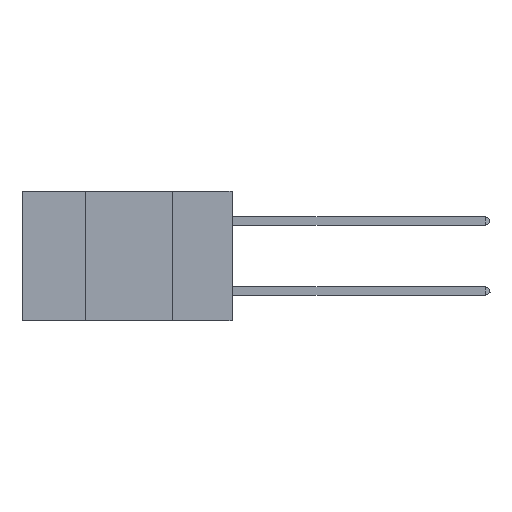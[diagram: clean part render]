
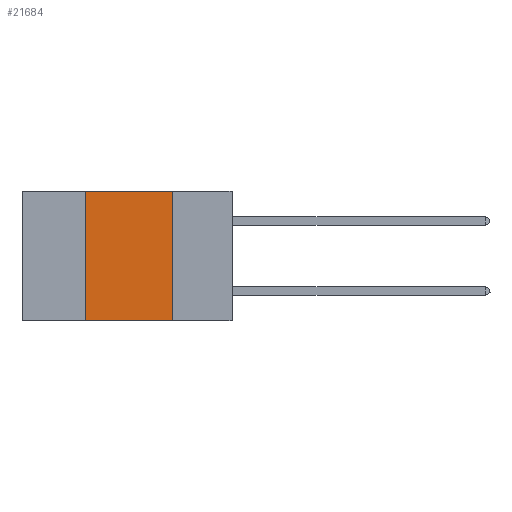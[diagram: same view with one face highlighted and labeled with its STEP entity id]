
A CAD part, left-side view. The second image highlights one B-rep face of the part: STEP entity #21684.
In plain terms, the highlighted planar face has unit normal (-1, 0, 0).
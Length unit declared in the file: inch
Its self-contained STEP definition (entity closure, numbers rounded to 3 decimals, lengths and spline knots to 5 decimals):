
#92 = CARTESIAN_POINT ( 'NONE',  ( 0., 0.42, 0. ) ) ;
#700 = AXIS2_PLACEMENT_3D ( 'NONE', #7568, #22101, #24284 ) ;
#1999 = DIRECTION ( 'NONE',  ( 0., -1., 0. ) ) ;
#3115 = EDGE_CURVE ( 'NONE', #4503, #23749, #26692, .T. ) ;
#3599 = EDGE_CURVE ( 'NONE', #7550, #9196, #25687, .T. ) ;
#3965 = EDGE_LOOP ( 'NONE', ( #4699, #14611, #3979, #21877 ) ) ;
#3979 = ORIENTED_EDGE ( 'NONE', *, *, #16165, .F. ) ;
#4019 = CARTESIAN_POINT ( 'NONE',  ( 0., 0.6, 0. ) ) ;
#4437 = VECTOR ( 'NONE', #5780, 39.37008 ) ;
#4503 = VERTEX_POINT ( 'NONE', #26522 ) ;
#4699 = ORIENTED_EDGE ( 'NONE', *, *, #23903, .F. ) ;
#5780 = DIRECTION ( 'NONE',  ( 0., 0., -1. ) ) ;
#7010 = CARTESIAN_POINT ( 'NONE',  ( 0., 0.17, 0. ) ) ;
#7550 = VERTEX_POINT ( 'NONE', #11514 ) ;
#7568 = CARTESIAN_POINT ( 'NONE',  ( 0., 0.6, 0. ) ) ;
#9196 = VERTEX_POINT ( 'NONE', #15745 ) ;
#11514 = CARTESIAN_POINT ( 'NONE',  ( 0., 0.42, -0.37 ) ) ;
#13509 = FACE_OUTER_BOUND ( 'NONE', #3965, .T. ) ;
#13911 = VECTOR ( 'NONE', #22919, 39.37008 ) ;
#14611 = ORIENTED_EDGE ( 'NONE', *, *, #3115, .F. ) ;
#15567 = VECTOR ( 'NONE', #1999, 39.37008 ) ;
#15745 = CARTESIAN_POINT ( 'NONE',  ( 0., 0.17, -0.37 ) ) ;
#16165 = EDGE_CURVE ( 'NONE', #7550, #4503, #25468, .T. ) ;
#17620 = CARTESIAN_POINT ( 'NONE',  ( 0., 0.6, -0.37 ) ) ;
#17866 = PLANE ( 'NONE',  #700 ) ;
#20934 = DIRECTION ( 'NONE',  ( 0., 0., 1. ) ) ;
#21684 = ADVANCED_FACE ( 'NONE', ( #13509 ), #17866, .F. ) ;
#21877 = ORIENTED_EDGE ( 'NONE', *, *, #3599, .T. ) ;
#22101 = DIRECTION ( 'NONE',  ( 1., 0., 0. ) ) ;
#22240 = VECTOR ( 'NONE', #20934, 39.37008 ) ;
#22919 = DIRECTION ( 'NONE',  ( 0., -1., 0. ) ) ;
#23749 = VERTEX_POINT ( 'NONE', #7010 ) ;
#23903 = EDGE_CURVE ( 'NONE', #23749, #9196, #24788, .T. ) ;
#24284 = DIRECTION ( 'NONE',  ( 0., 0., -1. ) ) ;
#24788 = LINE ( 'NONE', #26562, #4437 ) ;
#25468 = LINE ( 'NONE', #92, #22240 ) ;
#25687 = LINE ( 'NONE', #17620, #13911 ) ;
#26522 = CARTESIAN_POINT ( 'NONE',  ( 0., 0.42, 0. ) ) ;
#26562 = CARTESIAN_POINT ( 'NONE',  ( 0., 0.17, 0. ) ) ;
#26692 = LINE ( 'NONE', #4019, #15567 ) ;
